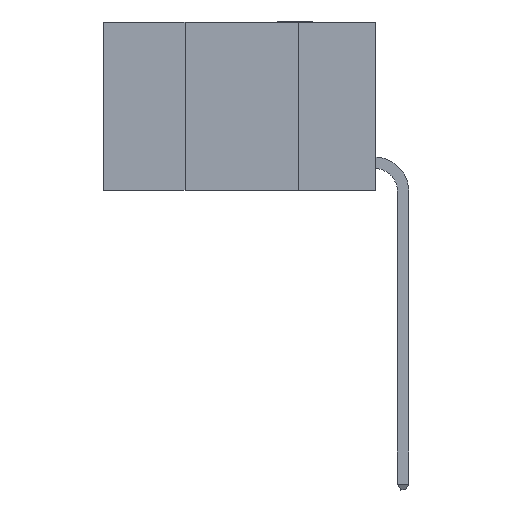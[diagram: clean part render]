
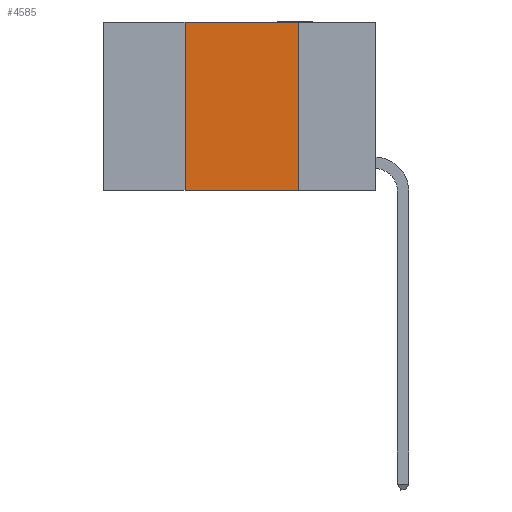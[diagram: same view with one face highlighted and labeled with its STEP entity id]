
A CAD part, left-side view. The second image highlights one B-rep face of the part: STEP entity #4585.
In plain terms, the highlighted planar face has unit normal (-1, 0, 0).
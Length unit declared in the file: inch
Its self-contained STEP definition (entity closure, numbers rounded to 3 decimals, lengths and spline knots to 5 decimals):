
#311 = VERTEX_POINT ( 'NONE', #7057 ) ;
#324 = LINE ( 'NONE', #9208, #7089 ) ;
#589 = DIRECTION ( 'NONE',  ( 0., -1., 0. ) ) ;
#592 = CARTESIAN_POINT ( 'NONE',  ( 0., 0.17, -0.37 ) ) ;
#886 = DIRECTION ( 'NONE',  ( 0., -1., 0. ) ) ;
#2403 = DIRECTION ( 'NONE',  ( 0., 0., -1. ) ) ;
#2855 = ORIENTED_EDGE ( 'NONE', *, *, #5834, .T. ) ;
#3274 = EDGE_LOOP ( 'NONE', ( #10948, #11152, #4225, #2855 ) ) ;
#3721 = EDGE_CURVE ( 'NONE', #311, #8992, #5966, .T. ) ;
#4141 = LINE ( 'NONE', #12926, #8130 ) ;
#4225 = ORIENTED_EDGE ( 'NONE', *, *, #13376, .F. ) ;
#4585 = ADVANCED_FACE ( 'NONE', ( #5711 ), #10128, .F. ) ;
#4890 = CARTESIAN_POINT ( 'NONE',  ( 0., 0.17, 0. ) ) ;
#5099 = DIRECTION ( 'NONE',  ( 0., 0., 1. ) ) ;
#5104 = VECTOR ( 'NONE', #9305, 39.37008 ) ;
#5687 = AXIS2_PLACEMENT_3D ( 'NONE', #13486, #12379, #2403 ) ;
#5711 = FACE_OUTER_BOUND ( 'NONE', #3274, .T. ) ;
#5797 = VERTEX_POINT ( 'NONE', #5872 ) ;
#5834 = EDGE_CURVE ( 'NONE', #5797, #8992, #324, .T. ) ;
#5872 = CARTESIAN_POINT ( 'NONE',  ( 0., 0.42, -0.37 ) ) ;
#5966 = LINE ( 'NONE', #4890, #5104 ) ;
#7057 = CARTESIAN_POINT ( 'NONE',  ( 0., 0.17, 0. ) ) ;
#7089 = VECTOR ( 'NONE', #886, 39.37008 ) ;
#7708 = EDGE_CURVE ( 'NONE', #9858, #311, #13910, .T. ) ;
#8130 = VECTOR ( 'NONE', #5099, 39.37008 ) ;
#8992 = VERTEX_POINT ( 'NONE', #592 ) ;
#9208 = CARTESIAN_POINT ( 'NONE',  ( 0., 0.6, -0.37 ) ) ;
#9305 = DIRECTION ( 'NONE',  ( 0., 0., -1. ) ) ;
#9858 = VERTEX_POINT ( 'NONE', #10458 ) ;
#10128 = PLANE ( 'NONE',  #5687 ) ;
#10458 = CARTESIAN_POINT ( 'NONE',  ( 0., 0.42, 0. ) ) ;
#10948 = ORIENTED_EDGE ( 'NONE', *, *, #3721, .F. ) ;
#11152 = ORIENTED_EDGE ( 'NONE', *, *, #7708, .F. ) ;
#11963 = VECTOR ( 'NONE', #589, 39.37008 ) ;
#12379 = DIRECTION ( 'NONE',  ( 1., 0., 0. ) ) ;
#12874 = CARTESIAN_POINT ( 'NONE',  ( 0., 0.6, 0. ) ) ;
#12926 = CARTESIAN_POINT ( 'NONE',  ( 0., 0.42, 0. ) ) ;
#13376 = EDGE_CURVE ( 'NONE', #5797, #9858, #4141, .T. ) ;
#13486 = CARTESIAN_POINT ( 'NONE',  ( 0., 0.6, 0. ) ) ;
#13910 = LINE ( 'NONE', #12874, #11963 ) ;
